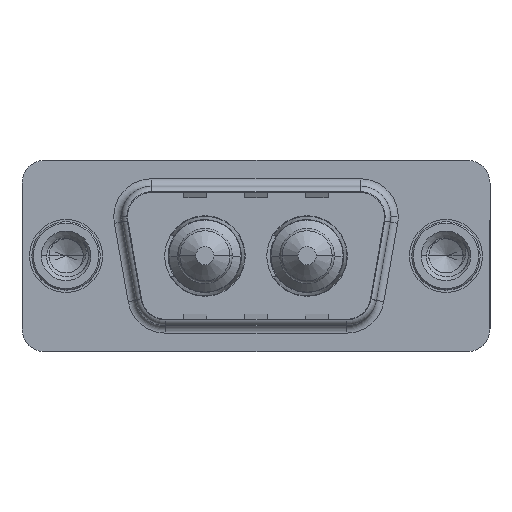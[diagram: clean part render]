
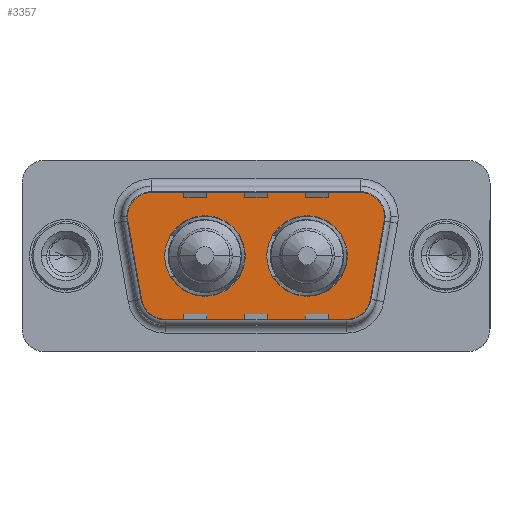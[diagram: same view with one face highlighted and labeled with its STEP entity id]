
A CAD part, top view. The second image highlights one B-rep face of the part: STEP entity #3357.
In plain terms, the highlighted planar face has unit normal (0, 0, 1).
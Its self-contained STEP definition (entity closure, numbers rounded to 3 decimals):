
#57 = DIRECTION ( 'NONE',  ( 0., 0., 1. ) ) ;
#98 = ORIENTED_EDGE ( 'NONE', *, *, #4002, .F. ) ;
#110 = CIRCLE ( 'NONE', #3783, 2. ) ;
#265 = DIRECTION ( 'NONE',  ( 1., 0., 0. ) ) ;
#406 = EDGE_CURVE ( 'NONE', #10227, #9444, #13086, .T. ) ;
#587 = CARTESIAN_POINT ( 'NONE',  ( 19.564, 2.9, 0. ) ) ;
#622 = EDGE_LOOP ( 'NONE', ( #98, #3641 ) ) ;
#724 = DIRECTION ( 'NONE',  ( 0., 0., 1. ) ) ;
#842 = DIRECTION ( 'NONE',  ( 0., 0., 1. ) ) ;
#934 = EDGE_CURVE ( 'NONE', #7299, #9277, #3370, .T. ) ;
#938 = EDGE_CURVE ( 'NONE', #2935, #7299, #3716, .T. ) ;
#977 = CARTESIAN_POINT ( 'NONE',  ( 21.534, 2.553, 0. ) ) ;
#1157 = CARTESIAN_POINT ( 'NONE',  ( 21.534, 2.553, 0. ) ) ;
#1438 = VERTEX_POINT ( 'NONE', #3630 ) ;
#1691 = EDGE_CURVE ( 'NONE', #12351, #1438, #9703, .T. ) ;
#1709 = EDGE_CURVE ( 'NONE', #12868, #11466, #11766, .T. ) ;
#1794 = CIRCLE ( 'NONE', #8084, 2. ) ;
#1940 = ORIENTED_EDGE ( 'NONE', *, *, #6847, .T. ) ;
#1954 = CARTESIAN_POINT ( 'NONE',  ( 15.86, 0., 0. ) ) ;
#2195 = VECTOR ( 'NONE', #12254, 1000. ) ;
#2228 = CARTESIAN_POINT ( 'NONE',  ( 3.466, 2.553, 0. ) ) ;
#2604 = EDGE_CURVE ( 'NONE', #11466, #12868, #12807, .T. ) ;
#2642 = ORIENTED_EDGE ( 'NONE', *, *, #1709, .F. ) ;
#2814 = CARTESIAN_POINT ( 'NONE',  ( 18.541, -2.9, 0. ) ) ;
#2883 = ORIENTED_EDGE ( 'NONE', *, *, #934, .T. ) ;
#2935 = VERTEX_POINT ( 'NONE', #1157 ) ;
#2990 = CIRCLE ( 'NONE', #9131, 2. ) ;
#3019 = DIRECTION ( 'NONE',  ( 1., 0., 0. ) ) ;
#3062 = AXIS2_PLACEMENT_3D ( 'NONE', #6960, #724, #8011 ) ;
#3063 = CARTESIAN_POINT ( 'NONE',  ( 9.14, 0., 0. ) ) ;
#3080 = VERTEX_POINT ( 'NONE', #5550 ) ;
#3226 = EDGE_LOOP ( 'NONE', ( #2642, #11355 ) ) ;
#3229 = CARTESIAN_POINT ( 'NONE',  ( 19.564, 4.9, 0. ) ) ;
#3357 = ADVANCED_FACE ( 'NONE', ( #11189, #5688, #8447 ), #12207, .T. ) ;
#3370 = CIRCLE ( 'NONE', #12642, 2. ) ;
#3440 = DIRECTION ( 'NONE',  ( 0., 0., 1. ) ) ;
#3630 = CARTESIAN_POINT ( 'NONE',  ( 18.51, 0., 0. ) ) ;
#3641 = ORIENTED_EDGE ( 'NONE', *, *, #1691, .F. ) ;
#3716 = CIRCLE ( 'NONE', #13334, 2. ) ;
#3783 = AXIS2_PLACEMENT_3D ( 'NONE', #2814, #10082, #3873 ) ;
#3865 = DIRECTION ( 'NONE',  ( 0., 0., 1. ) ) ;
#3873 = DIRECTION ( 'NONE',  ( 1., 0., 0. ) ) ;
#4002 = EDGE_CURVE ( 'NONE', #1438, #12351, #8413, .T. ) ;
#4004 = EDGE_CURVE ( 'NONE', #6289, #13319, #110, .T. ) ;
#4013 = ORIENTED_EDGE ( 'NONE', *, *, #938, .T. ) ;
#4110 = DIRECTION ( 'NONE',  ( 1., 0., 0. ) ) ;
#4380 = VECTOR ( 'NONE', #265, 1000. ) ;
#4402 = CARTESIAN_POINT ( 'NONE',  ( 18.541, -4.9, 0. ) ) ;
#4490 = CARTESIAN_POINT ( 'NONE',  ( 19.564, 2.9, 0. ) ) ;
#4866 = CARTESIAN_POINT ( 'NONE',  ( 3.466, 2.553, 0. ) ) ;
#5389 = EDGE_CURVE ( 'NONE', #13319, #2935, #6103, .T. ) ;
#5550 = CARTESIAN_POINT ( 'NONE',  ( 5.436, 4.9, 0. ) ) ;
#5688 = FACE_BOUND ( 'NONE', #3226, .T. ) ;
#5965 = DIRECTION ( 'NONE',  ( 0., 0., 1. ) ) ;
#6103 = LINE ( 'NONE', #977, #9205 ) ;
#6207 = CARTESIAN_POINT ( 'NONE',  ( 6.459, -4.9, 0. ) ) ;
#6289 = VERTEX_POINT ( 'NONE', #4402 ) ;
#6292 = CARTESIAN_POINT ( 'NONE',  ( 6.459, -2.9, 0. ) ) ;
#6813 = DIRECTION ( 'NONE',  ( -1., 0., 0. ) ) ;
#6847 = EDGE_CURVE ( 'NONE', #3080, #10227, #2990, .T. ) ;
#6954 = CARTESIAN_POINT ( 'NONE',  ( 13.21, 0., 0. ) ) ;
#6960 = CARTESIAN_POINT ( 'NONE',  ( 15.86, 0., 0. ) ) ;
#7299 = VERTEX_POINT ( 'NONE', #8240 ) ;
#7334 = DIRECTION ( 'NONE',  ( -1., 0., 0. ) ) ;
#7676 = CARTESIAN_POINT ( 'NONE',  ( 4.489, -3.247, 0. ) ) ;
#7743 = CARTESIAN_POINT ( 'NONE',  ( 6.49, 0., 0. ) ) ;
#7923 = VERTEX_POINT ( 'NONE', #6207 ) ;
#7956 = EDGE_CURVE ( 'NONE', #9444, #7923, #1794, .T. ) ;
#8011 = DIRECTION ( 'NONE',  ( 1., 0., 0. ) ) ;
#8084 = AXIS2_PLACEMENT_3D ( 'NONE', #6292, #57, #7334 ) ;
#8101 = ORIENTED_EDGE ( 'NONE', *, *, #406, .T. ) ;
#8126 = DIRECTION ( 'NONE',  ( 1., 0., 0. ) ) ;
#8240 = CARTESIAN_POINT ( 'NONE',  ( 21.564, 2.9, 0. ) ) ;
#8258 = CARTESIAN_POINT ( 'NONE',  ( 11.79, 0., 0. ) ) ;
#8413 = CIRCLE ( 'NONE', #3062, 2.65 ) ;
#8447 = FACE_OUTER_BOUND ( 'NONE', #9134, .T. ) ;
#8863 = EDGE_CURVE ( 'NONE', #7923, #6289, #12616, .T. ) ;
#9005 = DIRECTION ( 'NONE',  ( 0.174, -0.985, 0. ) ) ;
#9131 = AXIS2_PLACEMENT_3D ( 'NONE', #9672, #3440, #10686 ) ;
#9134 = EDGE_LOOP ( 'NONE', ( #10029, #12774, #4013, #2883, #9275, #1940, #8101, #9863, #11402 ) ) ;
#9137 = CARTESIAN_POINT ( 'NONE',  ( 18.541, -2.9, 0. ) ) ;
#9205 = VECTOR ( 'NONE', #13367, 1000. ) ;
#9224 = CARTESIAN_POINT ( 'NONE',  ( 5.436, 4.9, 0. ) ) ;
#9252 = DIRECTION ( 'NONE',  ( 0., 0., 1. ) ) ;
#9275 = ORIENTED_EDGE ( 'NONE', *, *, #12446, .T. ) ;
#9277 = VERTEX_POINT ( 'NONE', #3229 ) ;
#9396 = AXIS2_PLACEMENT_3D ( 'NONE', #1954, #9252, #3019 ) ;
#9444 = VERTEX_POINT ( 'NONE', #7676 ) ;
#9672 = CARTESIAN_POINT ( 'NONE',  ( 5.436, 2.9, 0. ) ) ;
#9703 = CIRCLE ( 'NONE', #9396, 2.65 ) ;
#9863 = ORIENTED_EDGE ( 'NONE', *, *, #7956, .T. ) ;
#10029 = ORIENTED_EDGE ( 'NONE', *, *, #4004, .T. ) ;
#10071 = DIRECTION ( 'NONE',  ( -1., 0., 0. ) ) ;
#10082 = DIRECTION ( 'NONE',  ( 0., 0., 1. ) ) ;
#10101 = AXIS2_PLACEMENT_3D ( 'NONE', #9137, #842, #8126 ) ;
#10227 = VERTEX_POINT ( 'NONE', #2228 ) ;
#10309 = DIRECTION ( 'NONE',  ( 0., 0., 1. ) ) ;
#10357 = VECTOR ( 'NONE', #9005, 1000. ) ;
#10487 = LINE ( 'NONE', #9224, #2195 ) ;
#10686 = DIRECTION ( 'NONE',  ( 1., 0., 0. ) ) ;
#11043 = DIRECTION ( 'NONE',  ( 0., 0., 1. ) ) ;
#11189 = FACE_BOUND ( 'NONE', #622, .T. ) ;
#11355 = ORIENTED_EDGE ( 'NONE', *, *, #2604, .F. ) ;
#11402 = ORIENTED_EDGE ( 'NONE', *, *, #8863, .T. ) ;
#11433 = AXIS2_PLACEMENT_3D ( 'NONE', #3063, #10309, #4110 ) ;
#11466 = VERTEX_POINT ( 'NONE', #7743 ) ;
#11636 = CARTESIAN_POINT ( 'NONE',  ( 6.459, -4.9, 0. ) ) ;
#11766 = CIRCLE ( 'NONE', #11433, 2.65 ) ;
#12144 = CARTESIAN_POINT ( 'NONE',  ( 9.14, 0., 0. ) ) ;
#12207 = PLANE ( 'NONE',  #10101 ) ;
#12224 = AXIS2_PLACEMENT_3D ( 'NONE', #12144, #5965, #13175 ) ;
#12254 = DIRECTION ( 'NONE',  ( -1., 0., 0. ) ) ;
#12351 = VERTEX_POINT ( 'NONE', #6954 ) ;
#12412 = CARTESIAN_POINT ( 'NONE',  ( 20.511, -3.247, 0. ) ) ;
#12446 = EDGE_CURVE ( 'NONE', #9277, #3080, #10487, .T. ) ;
#12616 = LINE ( 'NONE', #11636, #4380 ) ;
#12642 = AXIS2_PLACEMENT_3D ( 'NONE', #587, #11043, #6813 ) ;
#12774 = ORIENTED_EDGE ( 'NONE', *, *, #5389, .T. ) ;
#12807 = CIRCLE ( 'NONE', #12224, 2.65 ) ;
#12868 = VERTEX_POINT ( 'NONE', #8258 ) ;
#13086 = LINE ( 'NONE', #4866, #10357 ) ;
#13175 = DIRECTION ( 'NONE',  ( 1., 0., 0. ) ) ;
#13319 = VERTEX_POINT ( 'NONE', #12412 ) ;
#13334 = AXIS2_PLACEMENT_3D ( 'NONE', #4490, #3865, #10071 ) ;
#13367 = DIRECTION ( 'NONE',  ( 0.174, 0.985, 0. ) ) ;
